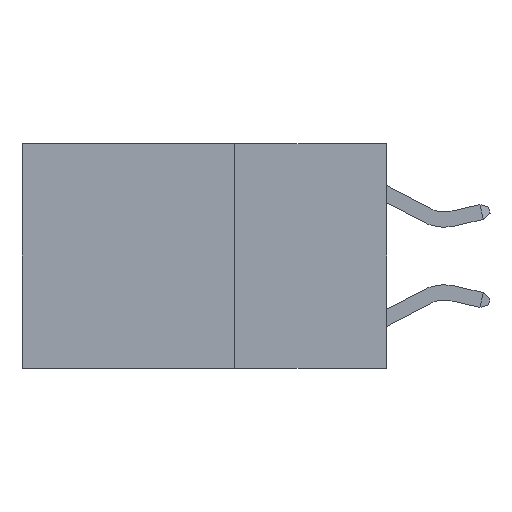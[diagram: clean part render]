
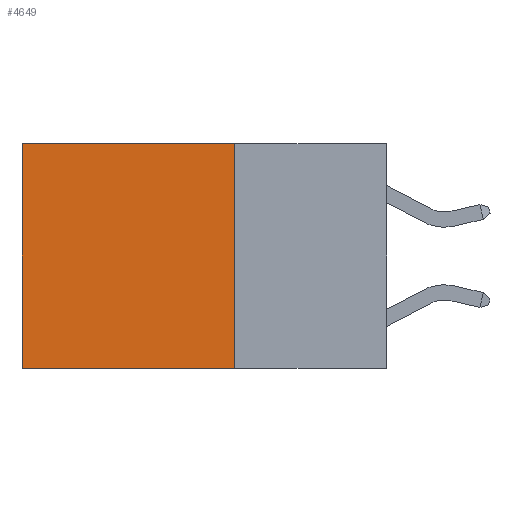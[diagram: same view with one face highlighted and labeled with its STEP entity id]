
A CAD part, left-side view. The second image highlights one B-rep face of the part: STEP entity #4649.
In plain terms, the highlighted planar face has unit normal (-1, 0, 0).
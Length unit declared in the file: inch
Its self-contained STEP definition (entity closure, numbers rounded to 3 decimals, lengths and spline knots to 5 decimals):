
#136 = CARTESIAN_POINT ( 'NONE',  ( 0.2625, 0.25, -0.37 ) ) ;
#804 = ORIENTED_EDGE ( 'NONE', *, *, #7972, .F. ) ;
#954 = CARTESIAN_POINT ( 'NONE',  ( 0.2625, 0.25, 0. ) ) ;
#1410 = CARTESIAN_POINT ( 'NONE',  ( 0.2625, 0.25, 0. ) ) ;
#2047 = VECTOR ( 'NONE', #10474, 39.37008 ) ;
#2299 = EDGE_LOOP ( 'NONE', ( #12174, #804, #5134, #2977 ) ) ;
#2315 = DIRECTION ( 'NONE',  ( 0., 0., -1. ) ) ;
#2977 = ORIENTED_EDGE ( 'NONE', *, *, #14516, .T. ) ;
#3081 = CARTESIAN_POINT ( 'NONE',  ( 0.2625, 0.6, 0. ) ) ;
#3934 = CARTESIAN_POINT ( 'NONE',  ( 0.2625, 0.6, 0. ) ) ;
#4419 = VECTOR ( 'NONE', #5299, 39.37008 ) ;
#4571 = DIRECTION ( 'NONE',  ( 1., 0., 0. ) ) ;
#4601 = EDGE_CURVE ( 'NONE', #14254, #7156, #11606, .T. ) ;
#4649 = ADVANCED_FACE ( 'NONE', ( #14131 ), #8163, .F. ) ;
#5134 = ORIENTED_EDGE ( 'NONE', *, *, #4601, .F. ) ;
#5299 = DIRECTION ( 'NONE',  ( 0., 0., -1. ) ) ;
#5869 = CARTESIAN_POINT ( 'NONE',  ( 0.2625, 0.25, -0.37 ) ) ;
#6035 = LINE ( 'NONE', #3934, #4419 ) ;
#6208 = VECTOR ( 'NONE', #7088, 39.37008 ) ;
#6232 = EDGE_CURVE ( 'NONE', #10022, #10241, #6035, .T. ) ;
#7088 = DIRECTION ( 'NONE',  ( 0., 1., 0. ) ) ;
#7156 = VERTEX_POINT ( 'NONE', #5869 ) ;
#7972 = EDGE_CURVE ( 'NONE', #7156, #10241, #8355, .T. ) ;
#8163 = PLANE ( 'NONE',  #8353 ) ;
#8353 = AXIS2_PLACEMENT_3D ( 'NONE', #10384, #4571, #2315 ) ;
#8355 = LINE ( 'NONE', #136, #2047 ) ;
#8779 = VECTOR ( 'NONE', #12379, 39.37008 ) ;
#10022 = VERTEX_POINT ( 'NONE', #3081 ) ;
#10241 = VERTEX_POINT ( 'NONE', #14686 ) ;
#10384 = CARTESIAN_POINT ( 'NONE',  ( 0.2625, 0.25, 0. ) ) ;
#10474 = DIRECTION ( 'NONE',  ( 0., 1., 0. ) ) ;
#11606 = LINE ( 'NONE', #12280, #8779 ) ;
#12174 = ORIENTED_EDGE ( 'NONE', *, *, #6232, .T. ) ;
#12280 = CARTESIAN_POINT ( 'NONE',  ( 0.2625, 0.25, 0. ) ) ;
#12379 = DIRECTION ( 'NONE',  ( 0., 0., -1. ) ) ;
#12482 = LINE ( 'NONE', #1410, #6208 ) ;
#14131 = FACE_OUTER_BOUND ( 'NONE', #2299, .T. ) ;
#14254 = VERTEX_POINT ( 'NONE', #954 ) ;
#14516 = EDGE_CURVE ( 'NONE', #14254, #10022, #12482, .T. ) ;
#14686 = CARTESIAN_POINT ( 'NONE',  ( 0.2625, 0.6, -0.37 ) ) ;
